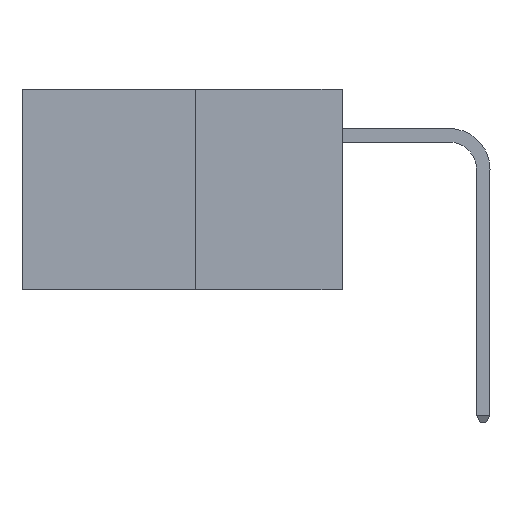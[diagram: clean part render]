
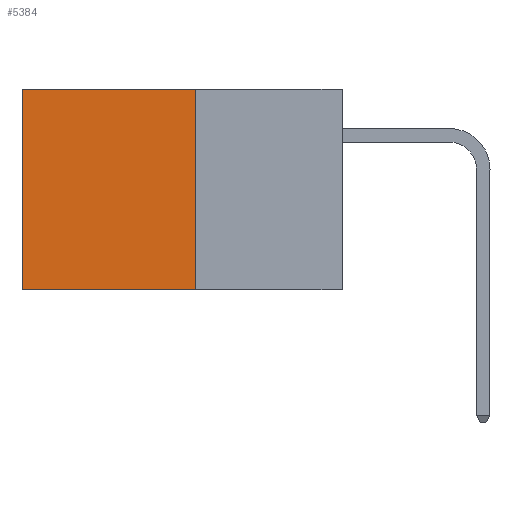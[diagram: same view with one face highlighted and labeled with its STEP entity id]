
A CAD part, left-side view. The second image highlights one B-rep face of the part: STEP entity #5384.
In plain terms, the highlighted planar face has unit normal (-1, 0, 0).
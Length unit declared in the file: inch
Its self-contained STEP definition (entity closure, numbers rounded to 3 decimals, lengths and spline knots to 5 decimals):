
#1402 = VECTOR ( 'NONE', #5573, 39.37008 ) ;
#2163 = DIRECTION ( 'NONE',  ( 0., 1., 0. ) ) ;
#2204 = CARTESIAN_POINT ( 'NONE',  ( 0.277, 0.27, -0.37 ) ) ;
#2427 = CARTESIAN_POINT ( 'NONE',  ( 0.277, 0.59, -0.37 ) ) ;
#3108 = VERTEX_POINT ( 'NONE', #4822 ) ;
#3734 = ORIENTED_EDGE ( 'NONE', *, *, #10767, .F. ) ;
#3924 = LINE ( 'NONE', #2427, #7878 ) ;
#4308 = PLANE ( 'NONE',  #9950 ) ;
#4599 = ORIENTED_EDGE ( 'NONE', *, *, #21774, .T. ) ;
#4822 = CARTESIAN_POINT ( 'NONE',  ( 0.277, 0.27, 0. ) ) ;
#5158 = CARTESIAN_POINT ( 'NONE',  ( 0.277, 0.59, -0.37 ) ) ;
#5183 = VERTEX_POINT ( 'NONE', #12263 ) ;
#5384 = ADVANCED_FACE ( 'NONE', ( #9291 ), #4308, .F. ) ;
#5573 = DIRECTION ( 'NONE',  ( 0., 0., -1. ) ) ;
#6018 = DIRECTION ( 'NONE',  ( 0., 0., -1. ) ) ;
#6048 = DIRECTION ( 'NONE',  ( 0., 1., 0. ) ) ;
#6419 = LINE ( 'NONE', #2204, #1402 ) ;
#7878 = VECTOR ( 'NONE', #14178, 39.37008 ) ;
#9291 = FACE_OUTER_BOUND ( 'NONE', #21072, .T. ) ;
#9950 = AXIS2_PLACEMENT_3D ( 'NONE', #14485, #16185, #6018 ) ;
#10075 = VECTOR ( 'NONE', #2163, 39.37008 ) ;
#10767 = EDGE_CURVE ( 'NONE', #5183, #16459, #20170, .T. ) ;
#11546 = ORIENTED_EDGE ( 'NONE', *, *, #15274, .F. ) ;
#12263 = CARTESIAN_POINT ( 'NONE',  ( 0.277, 0.27, -0.37 ) ) ;
#12301 = VERTEX_POINT ( 'NONE', #21864 ) ;
#14084 = CARTESIAN_POINT ( 'NONE',  ( 0.277, 0.27, -0.37 ) ) ;
#14178 = DIRECTION ( 'NONE',  ( 0., 0., -1. ) ) ;
#14485 = CARTESIAN_POINT ( 'NONE',  ( 0.277, 0.27, -0.37 ) ) ;
#15274 = EDGE_CURVE ( 'NONE', #3108, #5183, #6419, .T. ) ;
#15577 = VECTOR ( 'NONE', #6048, 39.37008 ) ;
#16185 = DIRECTION ( 'NONE',  ( 1., 0., 0. ) ) ;
#16459 = VERTEX_POINT ( 'NONE', #5158 ) ;
#17712 = ORIENTED_EDGE ( 'NONE', *, *, #20490, .T. ) ;
#19556 = CARTESIAN_POINT ( 'NONE',  ( 0.277, 0.27, 0. ) ) ;
#20095 = LINE ( 'NONE', #19556, #15577 ) ;
#20170 = LINE ( 'NONE', #14084, #10075 ) ;
#20490 = EDGE_CURVE ( 'NONE', #3108, #12301, #20095, .T. ) ;
#21072 = EDGE_LOOP ( 'NONE', ( #4599, #3734, #11546, #17712 ) ) ;
#21774 = EDGE_CURVE ( 'NONE', #12301, #16459, #3924, .T. ) ;
#21864 = CARTESIAN_POINT ( 'NONE',  ( 0.277, 0.59, 0. ) ) ;
